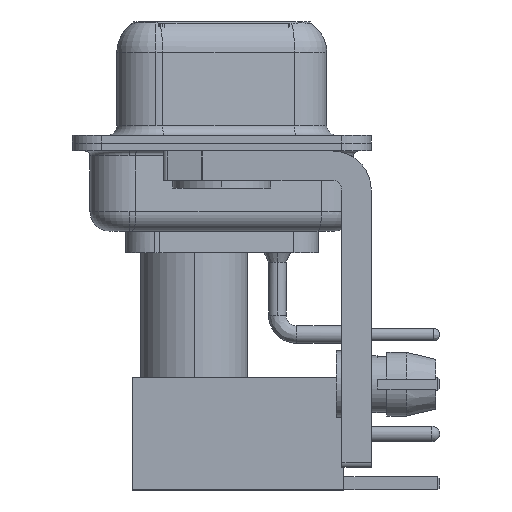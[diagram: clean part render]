
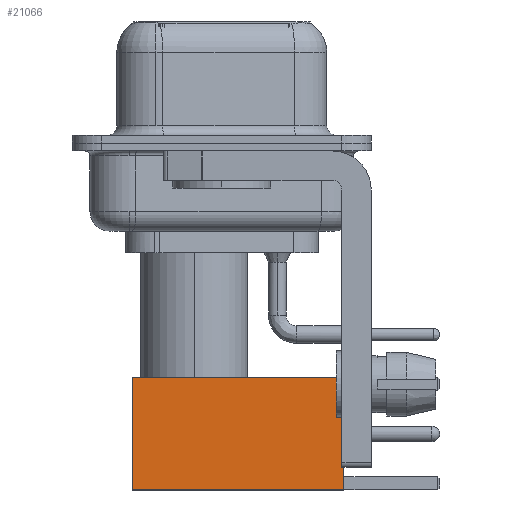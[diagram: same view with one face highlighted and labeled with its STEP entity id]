
A CAD part, left-side view. The second image highlights one B-rep face of the part: STEP entity #21066.
In plain terms, the highlighted face is planar.
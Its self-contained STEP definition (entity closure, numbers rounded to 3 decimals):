
#879 = DIRECTION ( 'NONE',  ( 0., 0., 1. ) ) ;
#994 = VERTEX_POINT ( 'NONE', #24818 ) ;
#1107 = LINE ( 'NONE', #12329, #7964 ) ;
#1329 = AXIS2_PLACEMENT_3D ( 'NONE', #3318, #22894, #879 ) ;
#1948 = DIRECTION ( 'NONE',  ( 0., 0., -1. ) ) ;
#2263 = ORIENTED_EDGE ( 'NONE', *, *, #12525, .T. ) ;
#3318 = CARTESIAN_POINT ( 'NONE',  ( 2.875, 2.875, 0. ) ) ;
#3443 = DIRECTION ( 'NONE',  ( 0., 0., -1. ) ) ;
#4676 = CARTESIAN_POINT ( 'NONE',  ( 2.875, 2.875, 0. ) ) ;
#5612 = PLANE ( 'NONE',  #1329 ) ;
#6604 = CARTESIAN_POINT ( 'NONE',  ( -2.875, 2.875, 10.82 ) ) ;
#7617 = FACE_OUTER_BOUND ( 'NONE', #19142, .T. ) ;
#7761 = CARTESIAN_POINT ( 'NONE',  ( -2.875, 2.875, 0. ) ) ;
#7964 = VECTOR ( 'NONE', #19077, 1000. ) ;
#8982 = LINE ( 'NONE', #4676, #10818 ) ;
#9285 = LINE ( 'NONE', #24963, #26291 ) ;
#9325 = VECTOR ( 'NONE', #3443, 1000. ) ;
#9375 = ORIENTED_EDGE ( 'NONE', *, *, #22942, .F. ) ;
#9712 = DIRECTION ( 'NONE',  ( -1., 0., 0. ) ) ;
#10098 = EDGE_CURVE ( 'NONE', #11794, #21386, #13959, .T. ) ;
#10526 = ORIENTED_EDGE ( 'NONE', *, *, #10098, .F. ) ;
#10818 = VECTOR ( 'NONE', #1948, 1000. ) ;
#11794 = VERTEX_POINT ( 'NONE', #6604 ) ;
#12329 = CARTESIAN_POINT ( 'NONE',  ( 0., 2.875, 10.82 ) ) ;
#12525 = EDGE_CURVE ( 'NONE', #15968, #21386, #9285, .T. ) ;
#13959 = LINE ( 'NONE', #7761, #9325 ) ;
#15968 = VERTEX_POINT ( 'NONE', #18149 ) ;
#16878 = ORIENTED_EDGE ( 'NONE', *, *, #17392, .T. ) ;
#17392 = EDGE_CURVE ( 'NONE', #994, #15968, #8982, .T. ) ;
#18149 = CARTESIAN_POINT ( 'NONE',  ( 2.875, 2.875, 0. ) ) ;
#19077 = DIRECTION ( 'NONE',  ( -1., 0., 0. ) ) ;
#19142 = EDGE_LOOP ( 'NONE', ( #16878, #2263, #10526, #9375 ) ) ;
#21066 = ADVANCED_FACE ( 'NONE', ( #7617 ), #5612, .T. ) ;
#21386 = VERTEX_POINT ( 'NONE', #26036 ) ;
#22894 = DIRECTION ( 'NONE',  ( 0., 1., 0. ) ) ;
#22942 = EDGE_CURVE ( 'NONE', #994, #11794, #1107, .T. ) ;
#24818 = CARTESIAN_POINT ( 'NONE',  ( 2.875, 2.875, 10.82 ) ) ;
#24963 = CARTESIAN_POINT ( 'NONE',  ( 0., 2.875, 0. ) ) ;
#26036 = CARTESIAN_POINT ( 'NONE',  ( -2.875, 2.875, 0. ) ) ;
#26291 = VECTOR ( 'NONE', #9712, 1000. ) ;
